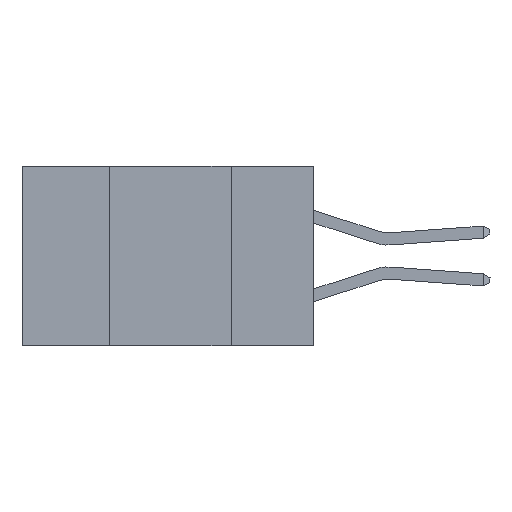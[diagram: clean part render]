
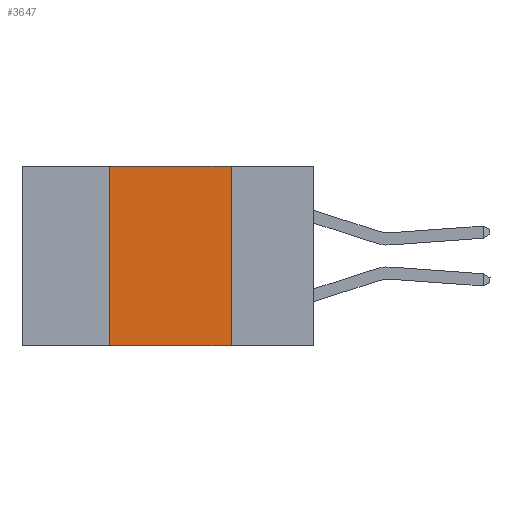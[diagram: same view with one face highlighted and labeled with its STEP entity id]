
A CAD part, left-side view. The second image highlights one B-rep face of the part: STEP entity #3647.
In plain terms, the highlighted planar face has unit normal (-1, 0, 0).
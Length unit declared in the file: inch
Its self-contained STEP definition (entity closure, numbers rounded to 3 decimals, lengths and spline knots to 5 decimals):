
#168 = EDGE_CURVE ( 'NONE', #9396, #4173, #468, .T. ) ;
#403 = VERTEX_POINT ( 'NONE', #6010 ) ;
#468 = LINE ( 'NONE', #1115, #4761 ) ;
#1115 = CARTESIAN_POINT ( 'NONE',  ( 0., 0.17, 0. ) ) ;
#1145 = DIRECTION ( 'NONE',  ( 0., 0., -1. ) ) ;
#1149 = CARTESIAN_POINT ( 'NONE',  ( 0., 0.42, 0. ) ) ;
#1324 = LINE ( 'NONE', #1149, #3034 ) ;
#1644 = EDGE_CURVE ( 'NONE', #403, #9396, #7842, .T. ) ;
#2324 = VERTEX_POINT ( 'NONE', #7839 ) ;
#2556 = DIRECTION ( 'NONE',  ( 0., 0., -1. ) ) ;
#2698 = DIRECTION ( 'NONE',  ( 1., 0., 0. ) ) ;
#3034 = VECTOR ( 'NONE', #10071, 39.37008 ) ;
#3635 = CARTESIAN_POINT ( 'NONE',  ( 0., 0.17, -0.37 ) ) ;
#3647 = ADVANCED_FACE ( 'NONE', ( #7109 ), #3684, .F. ) ;
#3684 = PLANE ( 'NONE',  #4887 ) ;
#3850 = LINE ( 'NONE', #9089, #8903 ) ;
#3996 = EDGE_LOOP ( 'NONE', ( #7430, #7348, #4512, #8800 ) ) ;
#4173 = VERTEX_POINT ( 'NONE', #3635 ) ;
#4512 = ORIENTED_EDGE ( 'NONE', *, *, #8611, .F. ) ;
#4761 = VECTOR ( 'NONE', #1145, 39.37008 ) ;
#4887 = AXIS2_PLACEMENT_3D ( 'NONE', #7386, #2698, #2556 ) ;
#4940 = DIRECTION ( 'NONE',  ( 0., -1., 0. ) ) ;
#6010 = CARTESIAN_POINT ( 'NONE',  ( 0., 0.42, 0. ) ) ;
#7109 = FACE_OUTER_BOUND ( 'NONE', #3996, .T. ) ;
#7262 = CARTESIAN_POINT ( 'NONE',  ( 0., 0.6, 0. ) ) ;
#7348 = ORIENTED_EDGE ( 'NONE', *, *, #1644, .F. ) ;
#7386 = CARTESIAN_POINT ( 'NONE',  ( 0., 0.6, 0. ) ) ;
#7430 = ORIENTED_EDGE ( 'NONE', *, *, #168, .F. ) ;
#7637 = EDGE_CURVE ( 'NONE', #2324, #4173, #3850, .T. ) ;
#7839 = CARTESIAN_POINT ( 'NONE',  ( 0., 0.42, -0.37 ) ) ;
#7842 = LINE ( 'NONE', #7262, #9575 ) ;
#8611 = EDGE_CURVE ( 'NONE', #2324, #403, #1324, .T. ) ;
#8800 = ORIENTED_EDGE ( 'NONE', *, *, #7637, .T. ) ;
#8903 = VECTOR ( 'NONE', #9856, 39.37008 ) ;
#9089 = CARTESIAN_POINT ( 'NONE',  ( 0., 0.6, -0.37 ) ) ;
#9396 = VERTEX_POINT ( 'NONE', #10083 ) ;
#9575 = VECTOR ( 'NONE', #4940, 39.37008 ) ;
#9856 = DIRECTION ( 'NONE',  ( 0., -1., 0. ) ) ;
#10071 = DIRECTION ( 'NONE',  ( 0., 0., 1. ) ) ;
#10083 = CARTESIAN_POINT ( 'NONE',  ( 0., 0.17, 0. ) ) ;
